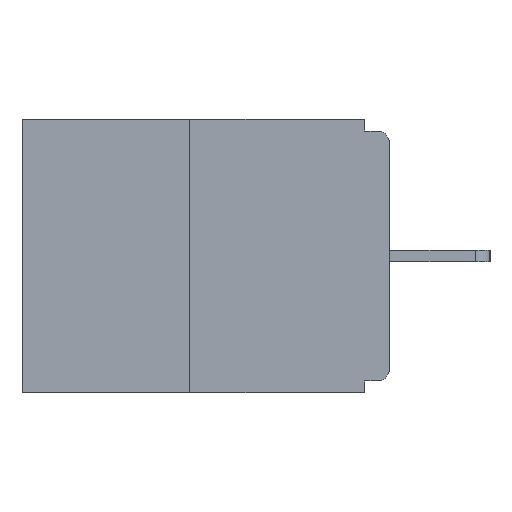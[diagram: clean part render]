
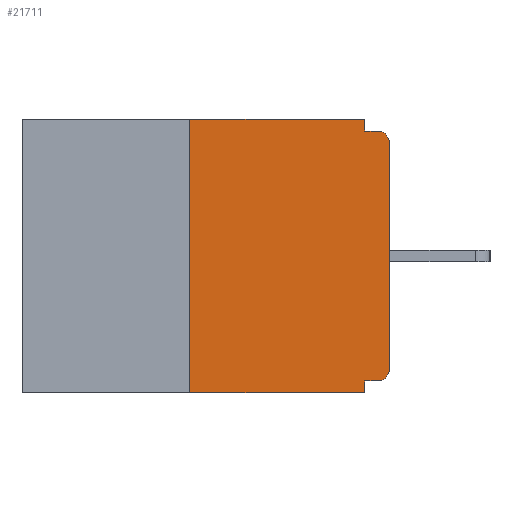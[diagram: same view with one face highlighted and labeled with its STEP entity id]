
A CAD part, left-side view. The second image highlights one B-rep face of the part: STEP entity #21711.
In plain terms, the highlighted planar face has unit normal (-1, 0, 0).
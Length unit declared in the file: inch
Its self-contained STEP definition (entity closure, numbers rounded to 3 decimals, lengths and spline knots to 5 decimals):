
#512 = ORIENTED_EDGE ( 'NONE', *, *, #19672, .F. ) ;
#525 = EDGE_CURVE ( 'NONE', #1529, #24532, #7573, .T. ) ;
#1448 = VECTOR ( 'NONE', #17754, 39.37008 ) ;
#1529 = VERTEX_POINT ( 'NONE', #14851 ) ;
#2733 = CARTESIAN_POINT ( 'NONE',  ( 0., 0.015, -0.313 ) ) ;
#2833 = VECTOR ( 'NONE', #3843, 39.37008 ) ;
#3707 = DIRECTION ( 'NONE',  ( 0., 0., -1. ) ) ;
#3730 = EDGE_CURVE ( 'NONE', #26639, #11499, #5792, .T. ) ;
#3843 = DIRECTION ( 'NONE',  ( 0., -1., 0. ) ) ;
#4439 = FACE_OUTER_BOUND ( 'NONE', #19939, .T. ) ;
#4609 = CARTESIAN_POINT ( 'NONE',  ( 0., 0.031, -0.343 ) ) ;
#4650 = DIRECTION ( 'NONE',  ( 0., 0., -1. ) ) ;
#4844 = CARTESIAN_POINT ( 'NONE',  ( 0., 0.031, -0.015 ) ) ;
#4959 = CARTESIAN_POINT ( 'NONE',  ( 0., 0., -0.313 ) ) ;
#5479 = VECTOR ( 'NONE', #26945, 39.37008 ) ;
#5560 = CARTESIAN_POINT ( 'NONE',  ( 0., 0.25, 0. ) ) ;
#5792 = LINE ( 'NONE', #9971, #15309 ) ;
#5817 = LINE ( 'NONE', #16646, #6808 ) ;
#6418 = VERTEX_POINT ( 'NONE', #4609 ) ;
#6433 = AXIS2_PLACEMENT_3D ( 'NONE', #25430, #19547, #13202 ) ;
#6595 = CARTESIAN_POINT ( 'NONE',  ( 0., 0.25, 0. ) ) ;
#6808 = VECTOR ( 'NONE', #18727, 39.37008 ) ;
#6900 = CIRCLE ( 'NONE', #7350, 0.015 ) ;
#7350 = AXIS2_PLACEMENT_3D ( 'NONE', #23824, #8962, #4650 ) ;
#7573 = CIRCLE ( 'NONE', #21779, 0.015 ) ;
#7682 = CARTESIAN_POINT ( 'NONE',  ( 0., 0.031, -0.328 ) ) ;
#7913 = CARTESIAN_POINT ( 'NONE',  ( 0., 0., 0. ) ) ;
#8368 = CARTESIAN_POINT ( 'NONE',  ( 0., 0.031, 0. ) ) ;
#8482 = PLANE ( 'NONE',  #6433 ) ;
#8525 = VERTEX_POINT ( 'NONE', #7682 ) ;
#8628 = ORIENTED_EDGE ( 'NONE', *, *, #11977, .F. ) ;
#8861 = DIRECTION ( 'NONE',  ( 0., 0., -1. ) ) ;
#8962 = DIRECTION ( 'NONE',  ( -1., 0., 0. ) ) ;
#9561 = CARTESIAN_POINT ( 'NONE',  ( 0., 0.25, -0.343 ) ) ;
#9672 = LINE ( 'NONE', #12293, #15348 ) ;
#9971 = CARTESIAN_POINT ( 'NONE',  ( 0., 0.031, 0. ) ) ;
#9995 = VERTEX_POINT ( 'NONE', #9561 ) ;
#10086 = DIRECTION ( 'NONE',  ( 0., -1., 0. ) ) ;
#11205 = DIRECTION ( 'NONE',  ( -1., 0., 0. ) ) ;
#11499 = VERTEX_POINT ( 'NONE', #4844 ) ;
#11607 = VECTOR ( 'NONE', #16082, 39.37008 ) ;
#11664 = EDGE_CURVE ( 'NONE', #18195, #26639, #14389, .T. ) ;
#11714 = ORIENTED_EDGE ( 'NONE', *, *, #19465, .F. ) ;
#11977 = EDGE_CURVE ( 'NONE', #8525, #6418, #17420, .T. ) ;
#12293 = CARTESIAN_POINT ( 'NONE',  ( 0., 0., -0.015 ) ) ;
#12440 = CARTESIAN_POINT ( 'NONE',  ( 0., 0.015, -0.015 ) ) ;
#12882 = ORIENTED_EDGE ( 'NONE', *, *, #525, .T. ) ;
#13202 = DIRECTION ( 'NONE',  ( 0., 0., -1. ) ) ;
#13258 = VERTEX_POINT ( 'NONE', #12440 ) ;
#14289 = LINE ( 'NONE', #7913, #11607 ) ;
#14389 = LINE ( 'NONE', #24543, #2833 ) ;
#14851 = CARTESIAN_POINT ( 'NONE',  ( 0., 0.015, -0.328 ) ) ;
#15309 = VECTOR ( 'NONE', #3707, 39.37008 ) ;
#15348 = VECTOR ( 'NONE', #10086, 39.37008 ) ;
#16082 = DIRECTION ( 'NONE',  ( 0., 0., 1. ) ) ;
#16628 = ORIENTED_EDGE ( 'NONE', *, *, #3730, .F. ) ;
#16646 = CARTESIAN_POINT ( 'NONE',  ( 0., 0.46, -0.343 ) ) ;
#17420 = LINE ( 'NONE', #23838, #22341 ) ;
#17724 = EDGE_CURVE ( 'NONE', #24532, #21063, #14289, .T. ) ;
#17754 = DIRECTION ( 'NONE',  ( 0., 1., 0. ) ) ;
#18195 = VERTEX_POINT ( 'NONE', #6595 ) ;
#18307 = ORIENTED_EDGE ( 'NONE', *, *, #19612, .T. ) ;
#18727 = DIRECTION ( 'NONE',  ( 0., -1., 0. ) ) ;
#18906 = CARTESIAN_POINT ( 'NONE',  ( 0., 0., -0.03 ) ) ;
#19077 = ORIENTED_EDGE ( 'NONE', *, *, #17724, .T. ) ;
#19099 = ORIENTED_EDGE ( 'NONE', *, *, #23752, .T. ) ;
#19465 = EDGE_CURVE ( 'NONE', #1529, #8525, #19985, .T. ) ;
#19547 = DIRECTION ( 'NONE',  ( 1., 0., 0. ) ) ;
#19612 = EDGE_CURVE ( 'NONE', #9995, #6418, #5817, .T. ) ;
#19622 = ORIENTED_EDGE ( 'NONE', *, *, #11664, .F. ) ;
#19672 = EDGE_CURVE ( 'NONE', #9995, #18195, #24588, .T. ) ;
#19939 = EDGE_LOOP ( 'NONE', ( #19622, #512, #18307, #8628, #11714, #12882, #19077, #19099, #22109, #16628 ) ) ;
#19985 = LINE ( 'NONE', #22089, #1448 ) ;
#21063 = VERTEX_POINT ( 'NONE', #18906 ) ;
#21618 = DIRECTION ( 'NONE',  ( 0., 0., -1. ) ) ;
#21711 = ADVANCED_FACE ( 'NONE', ( #4439 ), #8482, .F. ) ;
#21779 = AXIS2_PLACEMENT_3D ( 'NONE', #2733, #11205, #8861 ) ;
#22089 = CARTESIAN_POINT ( 'NONE',  ( 0., 0., -0.328 ) ) ;
#22109 = ORIENTED_EDGE ( 'NONE', *, *, #22380, .F. ) ;
#22341 = VECTOR ( 'NONE', #21618, 39.37008 ) ;
#22380 = EDGE_CURVE ( 'NONE', #11499, #13258, #9672, .T. ) ;
#23752 = EDGE_CURVE ( 'NONE', #21063, #13258, #6900, .T. ) ;
#23824 = CARTESIAN_POINT ( 'NONE',  ( 0., 0.015, -0.03 ) ) ;
#23838 = CARTESIAN_POINT ( 'NONE',  ( 0., 0.031, -0.343 ) ) ;
#24532 = VERTEX_POINT ( 'NONE', #4959 ) ;
#24543 = CARTESIAN_POINT ( 'NONE',  ( 0., 0.46, 0. ) ) ;
#24588 = LINE ( 'NONE', #5560, #5479 ) ;
#25430 = CARTESIAN_POINT ( 'NONE',  ( 0., 0.46, 0. ) ) ;
#26639 = VERTEX_POINT ( 'NONE', #8368 ) ;
#26945 = DIRECTION ( 'NONE',  ( 0., 0., 1. ) ) ;
